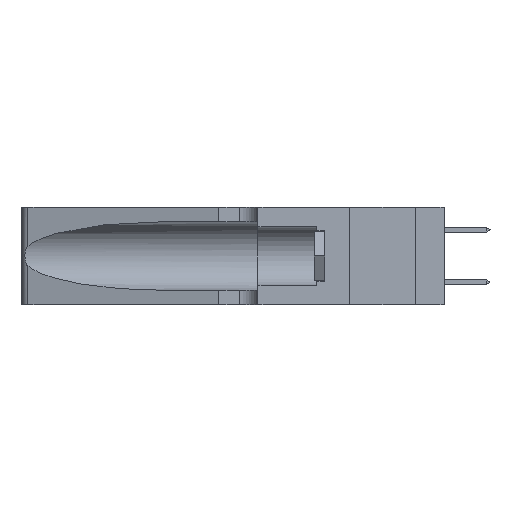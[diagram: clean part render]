
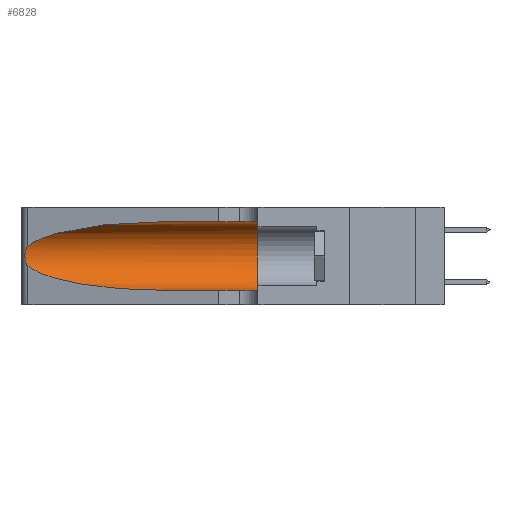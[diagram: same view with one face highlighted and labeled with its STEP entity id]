
A CAD part, left-side view. The second image highlights one B-rep face of the part: STEP entity #6828.
In plain terms, the highlighted cylindrical face has radius 3.308 mm (diameter 6.617 mm), a partial arc.
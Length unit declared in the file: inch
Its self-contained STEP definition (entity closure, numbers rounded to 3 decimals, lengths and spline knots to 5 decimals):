
#1082 = CARTESIAN_POINT ( 'NONE',  ( 0.1305, 0.35, 0.05475 ) ) ;
#1186 = AXIS2_PLACEMENT_3D ( 'NONE', #34761, #2963, #37955 ) ;
#2546 = ORIENTED_EDGE ( 'NONE', *, *, #20605, .T. ) ;
#2726 = EDGE_CURVE ( 'NONE', #40042, #22716, #6680, .T. ) ;
#2892 = CARTESIAN_POINT ( 'NONE',  ( 0.18966, 0.96281, 0.31525 ) ) ;
#2963 = DIRECTION ( 'NONE',  ( 0., 1., 0. ) ) ;
#5249 = DIRECTION ( 'NONE',  ( 0., -1., 0. ) ) ;
#5570 = CARTESIAN_POINT ( 'NONE',  ( 0.25789, 1.23486, 0.15765 ) ) ;
#6371 = ORIENTED_EDGE ( 'NONE', *, *, #37269, .T. ) ;
#6680 = B_SPLINE_CURVE_WITH_KNOTS ( 'NONE', 3,
 ( #40936, #31608, #15029, #15435, #37324, #40532, #21431, #34421, #21845, #24647, #5570, #12223, #15171, #34571 ),
 .UNSPECIFIED., .F., .F.,
 ( 4, 2, 2, 2, 2, 2, 4 ),
 ( 0., 0.00027, 0.00053, 0.00107, 0.0016, 0.00187, 0.00214 ),
 .UNSPECIFIED. ) ;
#6828 = ADVANCED_FACE ( 'NONE', ( #26156 ), #30638, .F. ) ;
#7361 = EDGE_LOOP ( 'NONE', ( #6371, #29748, #2546, #30114, #24001, #19992 ) ) ;
#7747 = CARTESIAN_POINT ( 'NONE',  ( 0.1305, 0.72297, 0.05475 ) ) ;
#9229 = EDGE_CURVE ( 'NONE', #9843, #36279, #20309, .T. ) ;
#9843 = VERTEX_POINT ( 'NONE', #7747 ) ;
#11021 = CARTESIAN_POINT ( 'NONE',  ( 0.25487, 1.22718, 0.14631 ) ) ;
#12223 = CARTESIAN_POINT ( 'NONE',  ( 0.25639, 1.23186, 0.15144 ) ) ;
#12497 = CARTESIAN_POINT ( 'NONE',  ( 0.25487, 1.22718, 0.22369 ) ) ;
#15029 = CARTESIAN_POINT ( 'NONE',  ( 0.25639, 1.23184, 0.21858 ) ) ;
#15171 = CARTESIAN_POINT ( 'NONE',  ( 0.25555, 1.22993, 0.14849 ) ) ;
#15435 = CARTESIAN_POINT ( 'NONE',  ( 0.25787, 1.23484, 0.2124 ) ) ;
#15729 = CARTESIAN_POINT ( 'NONE',  ( 0.1305, 0.72297, 0.31525 ) ) ;
#18313 = AXIS2_PLACEMENT_3D ( 'NONE', #24337, #5249, #21402 ) ;
#18415 =( BOUNDED_CURVE ( )  B_SPLINE_CURVE ( 3, ( #18659, #34576, #37745, #18508 ),
 .UNSPECIFIED., .F., .T. ) 
 B_SPLINE_CURVE_WITH_KNOTS ( ( 4, 4 ),
 ( 3.44316, 4.71239 ),
 .UNSPECIFIED. ) 
 CURVE ( )  GEOMETRIC_REPRESENTATION_ITEM ( )  RATIONAL_B_SPLINE_CURVE ( ( 1., 0.87, 0.87, 1. ) ) 
 REPRESENTATION_ITEM ( '' )  );
#18508 = CARTESIAN_POINT ( 'NONE',  ( 0.1305, 0.72297, 0.05475 ) ) ;
#18659 = CARTESIAN_POINT ( 'NONE',  ( 0.25487, 1.22718, 0.14631 ) ) ;
#19992 = ORIENTED_EDGE ( 'NONE', *, *, #32836, .F. ) ;
#20309 = LINE ( 'NONE', #23868, #36294 ) ;
#20605 = EDGE_CURVE ( 'NONE', #22716, #9843, #18415, .T. ) ;
#20799 = DIRECTION ( 'NONE',  ( 0., -1., 0. ) ) ;
#21402 = DIRECTION ( 'NONE',  ( 0., 0., -1. ) ) ;
#21431 = CARTESIAN_POINT ( 'NONE',  ( 0.26075, 1.23896, 0.19203 ) ) ;
#21845 = CARTESIAN_POINT ( 'NONE',  ( 0.26017, 1.23833, 0.17102 ) ) ;
#21975 = CARTESIAN_POINT ( 'NONE',  ( 0.1305, 0.72297, 0.31525 ) ) ;
#22092 = VERTEX_POINT ( 'NONE', #15729 ) ;
#22568 = CIRCLE ( 'NONE', #1186, 0.13025 ) ;
#22716 = VERTEX_POINT ( 'NONE', #11021 ) ;
#23868 = CARTESIAN_POINT ( 'NONE',  ( 0.1305, 1.61858, 0.05475 ) ) ;
#24001 = ORIENTED_EDGE ( 'NONE', *, *, #28684, .F. ) ;
#24252 = LINE ( 'NONE', #39759, #24771 ) ;
#24337 = CARTESIAN_POINT ( 'NONE',  ( 0.1305, 1.61858, 0.185 ) ) ;
#24647 = CARTESIAN_POINT ( 'NONE',  ( 0.25856, 1.23593, 0.16098 ) ) ;
#24771 = VECTOR ( 'NONE', #27250, 39.37008 ) ;
#25360 = CARTESIAN_POINT ( 'NONE',  ( 0.1305, 0.35, 0.31525 ) ) ;
#26156 = FACE_OUTER_BOUND ( 'NONE', #7361, .T. ) ;
#27250 = DIRECTION ( 'NONE',  ( 0., -1., 0. ) ) ;
#28684 = EDGE_CURVE ( 'NONE', #36732, #36279, #22568, .T. ) ;
#29748 = ORIENTED_EDGE ( 'NONE', *, *, #2726, .T. ) ;
#30114 = ORIENTED_EDGE ( 'NONE', *, *, #9229, .T. ) ;
#30638 = CYLINDRICAL_SURFACE ( 'NONE', #18313, 0.13025 ) ;
#31608 = CARTESIAN_POINT ( 'NONE',  ( 0.25555, 1.22994, 0.2215 ) ) ;
#32836 = EDGE_CURVE ( 'NONE', #22092, #36732, #24252, .T. ) ;
#34421 = CARTESIAN_POINT ( 'NONE',  ( 0.26075, 1.23896, 0.178 ) ) ;
#34571 = CARTESIAN_POINT ( 'NONE',  ( 0.25487, 1.22718, 0.14631 ) ) ;
#34576 = CARTESIAN_POINT ( 'NONE',  ( 0.2373, 1.15595, 0.08982 ) ) ;
#34761 = CARTESIAN_POINT ( 'NONE',  ( 0.1305, 0.35, 0.185 ) ) ;
#36279 = VERTEX_POINT ( 'NONE', #1082 ) ;
#36294 = VECTOR ( 'NONE', #20799, 39.37008 ) ;
#36732 = VERTEX_POINT ( 'NONE', #25360 ) ;
#37074 =( BOUNDED_CURVE ( )  B_SPLINE_CURVE ( 3, ( #21975, #2892, #40776, #12497 ),
 .UNSPECIFIED., .F., .F. ) 
 B_SPLINE_CURVE_WITH_KNOTS ( ( 4, 4 ),
 ( 1.5708, 2.84003 ),
 .UNSPECIFIED. ) 
 CURVE ( )  GEOMETRIC_REPRESENTATION_ITEM ( )  RATIONAL_B_SPLINE_CURVE ( ( 1., 0.87, 0.87, 1. ) ) 
 REPRESENTATION_ITEM ( '' )  );
#37269 = EDGE_CURVE ( 'NONE', #22092, #40042, #37074, .T. ) ;
#37324 = CARTESIAN_POINT ( 'NONE',  ( 0.25854, 1.2359, 0.20912 ) ) ;
#37745 = CARTESIAN_POINT ( 'NONE',  ( 0.18966, 0.96281, 0.05475 ) ) ;
#37955 = DIRECTION ( 'NONE',  ( 0., 0., 1. ) ) ;
#39759 = CARTESIAN_POINT ( 'NONE',  ( 0.1305, 1.61858, 0.31525 ) ) ;
#40042 = VERTEX_POINT ( 'NONE', #40392 ) ;
#40392 = CARTESIAN_POINT ( 'NONE',  ( 0.25487, 1.22718, 0.22369 ) ) ;
#40532 = CARTESIAN_POINT ( 'NONE',  ( 0.26018, 1.23835, 0.19895 ) ) ;
#40776 = CARTESIAN_POINT ( 'NONE',  ( 0.2373, 1.15595, 0.28018 ) ) ;
#40936 = CARTESIAN_POINT ( 'NONE',  ( 0.25487, 1.22718, 0.22369 ) ) ;
